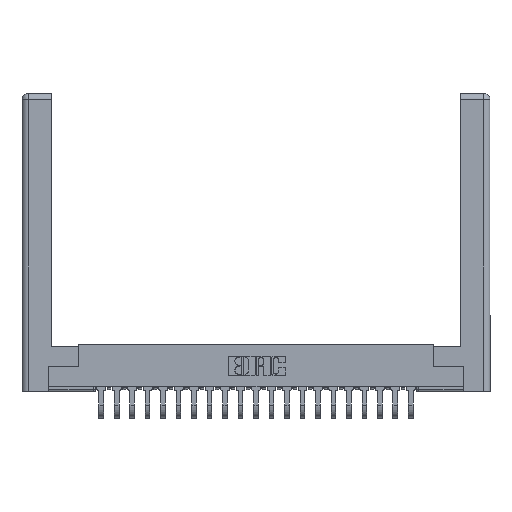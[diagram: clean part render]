
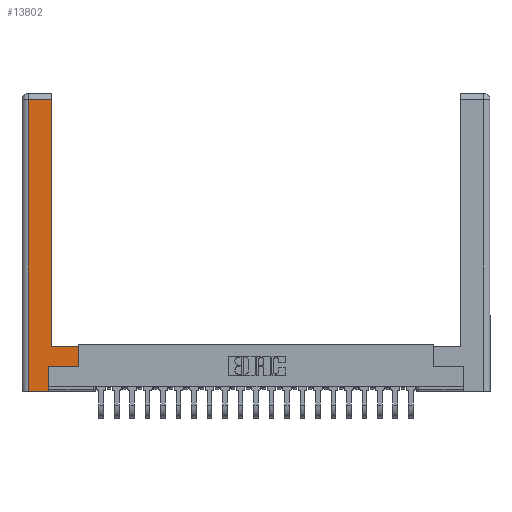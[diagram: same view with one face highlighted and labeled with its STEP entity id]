
A CAD part, top view. The second image highlights one B-rep face of the part: STEP entity #13802.
In plain terms, the highlighted planar face has unit normal (0, 0, 1).
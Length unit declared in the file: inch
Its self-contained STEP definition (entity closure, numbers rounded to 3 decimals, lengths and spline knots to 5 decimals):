
#8 = LINE ( 'NONE', #5669, #16643 ) ;
#221 = DIRECTION ( 'NONE',  ( 0., 0., -1. ) ) ;
#309 = LINE ( 'NONE', #18647, #17017 ) ;
#468 = PLANE ( 'NONE',  #6848 ) ;
#738 = CARTESIAN_POINT ( 'NONE',  ( 0.295, 2.94, 0. ) ) ;
#1012 = LINE ( 'NONE', #6445, #17732 ) ;
#1078 = VERTEX_POINT ( 'NONE', #9503 ) ;
#1393 = ORIENTED_EDGE ( 'NONE', *, *, #15722, .T. ) ;
#1961 = ORIENTED_EDGE ( 'NONE', *, *, #20674, .T. ) ;
#2219 = LINE ( 'NONE', #21819, #15437 ) ;
#2379 = DIRECTION ( 'NONE',  ( -1., 0., 0. ) ) ;
#2382 = CARTESIAN_POINT ( 'NONE',  ( 0.265, 0., 0. ) ) ;
#2810 = VERTEX_POINT ( 'NONE', #20275 ) ;
#3196 = CARTESIAN_POINT ( 'NONE',  ( 0.295, 3., 0. ) ) ;
#3238 = EDGE_CURVE ( 'NONE', #5725, #9115, #4492, .T. ) ;
#3320 = DIRECTION ( 'NONE',  ( -1., 0., 0. ) ) ;
#4492 = LINE ( 'NONE', #3196, #16894 ) ;
#4776 = VECTOR ( 'NONE', #5997, 39.37008 ) ;
#5529 = LINE ( 'NONE', #2382, #4776 ) ;
#5669 = CARTESIAN_POINT ( 'NONE',  ( 0.295, 0.45, 0. ) ) ;
#5725 = VERTEX_POINT ( 'NONE', #19936 ) ;
#5754 = DIRECTION ( 'NONE',  ( 0., 1., 0. ) ) ;
#5997 = DIRECTION ( 'NONE',  ( 1., 0., 0. ) ) ;
#6372 = EDGE_CURVE ( 'NONE', #9115, #1078, #23158, .T. ) ;
#6445 = CARTESIAN_POINT ( 'NONE',  ( 0.265, 0.245, 0. ) ) ;
#6848 = AXIS2_PLACEMENT_3D ( 'NONE', #20312, #221, #2379 ) ;
#7841 = ORIENTED_EDGE ( 'NONE', *, *, #19887, .T. ) ;
#8353 = CARTESIAN_POINT ( 'NONE',  ( 0.565, 0.245, 0. ) ) ;
#8424 = VERTEX_POINT ( 'NONE', #17672 ) ;
#8732 = DIRECTION ( 'NONE',  ( -1., 0., 0. ) ) ;
#9115 = VERTEX_POINT ( 'NONE', #738 ) ;
#9503 = CARTESIAN_POINT ( 'NONE',  ( 0.0615, 2.94, 0. ) ) ;
#9850 = CARTESIAN_POINT ( 'NONE',  ( 0.565, 0.45, 0. ) ) ;
#10346 = VERTEX_POINT ( 'NONE', #9850 ) ;
#11151 = VERTEX_POINT ( 'NONE', #14975 ) ;
#11346 = ORIENTED_EDGE ( 'NONE', *, *, #19974, .T. ) ;
#11513 = ORIENTED_EDGE ( 'NONE', *, *, #17368, .T. ) ;
#12060 = CARTESIAN_POINT ( 'NONE',  ( 0.0615, 2.94, 0. ) ) ;
#12468 = EDGE_CURVE ( 'NONE', #10346, #5725, #8, .T. ) ;
#13573 = VECTOR ( 'NONE', #8732, 39.37008 ) ;
#13660 = DIRECTION ( 'NONE',  ( 0., 1., 0. ) ) ;
#13802 = ADVANCED_FACE ( 'NONE', ( #16434 ), #468, .F. ) ;
#14127 = VERTEX_POINT ( 'NONE', #8353 ) ;
#14975 = CARTESIAN_POINT ( 'NONE',  ( 0.265, 0.245, 0. ) ) ;
#15224 = CARTESIAN_POINT ( 'NONE',  ( 0.565, 0.245, 0. ) ) ;
#15437 = VECTOR ( 'NONE', #18283, 39.37008 ) ;
#15722 = EDGE_CURVE ( 'NONE', #8424, #11151, #1012, .T. ) ;
#16434 = FACE_OUTER_BOUND ( 'NONE', #19544, .T. ) ;
#16643 = VECTOR ( 'NONE', #3320, 39.37008 ) ;
#16894 = VECTOR ( 'NONE', #22467, 39.37008 ) ;
#17017 = VECTOR ( 'NONE', #5754, 39.37008 ) ;
#17368 = EDGE_CURVE ( 'NONE', #14127, #10346, #309, .T. ) ;
#17672 = CARTESIAN_POINT ( 'NONE',  ( 0.265, 0., 0. ) ) ;
#17732 = VECTOR ( 'NONE', #13660, 39.37008 ) ;
#18032 = ORIENTED_EDGE ( 'NONE', *, *, #3238, .T. ) ;
#18283 = DIRECTION ( 'NONE',  ( 0., -1., 0. ) ) ;
#18647 = CARTESIAN_POINT ( 'NONE',  ( 0.565, 0.45, 0. ) ) ;
#18972 = ORIENTED_EDGE ( 'NONE', *, *, #6372, .T. ) ;
#19544 = EDGE_LOOP ( 'NONE', ( #18032, #18972, #7841, #1961, #1393, #11346, #11513, #22991 ) ) ;
#19887 = EDGE_CURVE ( 'NONE', #1078, #2810, #2219, .T. ) ;
#19936 = CARTESIAN_POINT ( 'NONE',  ( 0.295, 0.45, 0. ) ) ;
#19974 = EDGE_CURVE ( 'NONE', #11151, #14127, #22641, .T. ) ;
#20275 = CARTESIAN_POINT ( 'NONE',  ( 0.0615, 0., 0. ) ) ;
#20312 = CARTESIAN_POINT ( 'NONE',  ( 0., 0., 0. ) ) ;
#20674 = EDGE_CURVE ( 'NONE', #2810, #8424, #5529, .T. ) ;
#21819 = CARTESIAN_POINT ( 'NONE',  ( 0.0615, 0., 0. ) ) ;
#22467 = DIRECTION ( 'NONE',  ( 0., 1., 0. ) ) ;
#22519 = DIRECTION ( 'NONE',  ( 1., 0., 0. ) ) ;
#22641 = LINE ( 'NONE', #15224, #23315 ) ;
#22991 = ORIENTED_EDGE ( 'NONE', *, *, #12468, .T. ) ;
#23158 = LINE ( 'NONE', #12060, #13573 ) ;
#23315 = VECTOR ( 'NONE', #22519, 39.37008 ) ;
